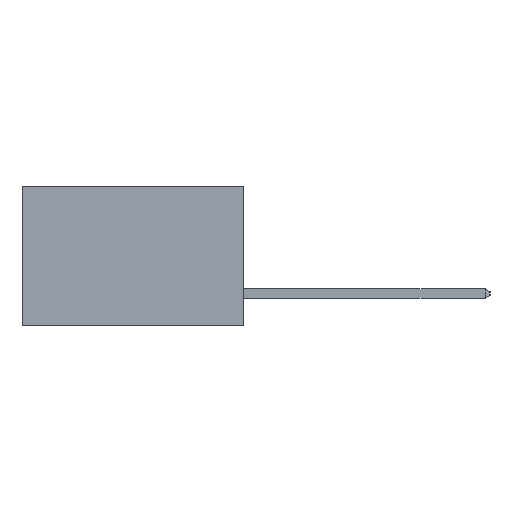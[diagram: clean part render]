
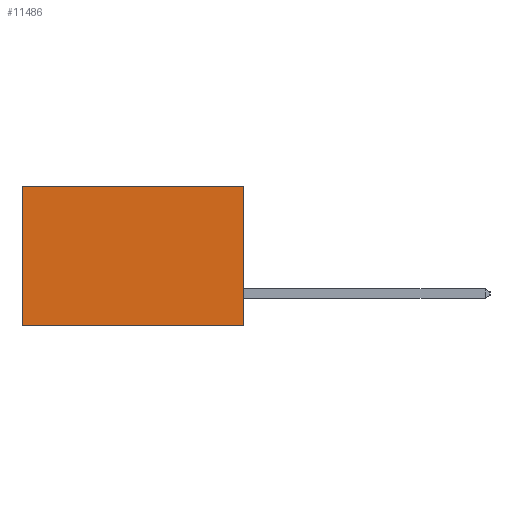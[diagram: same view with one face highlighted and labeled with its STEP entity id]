
A CAD part, left-side view. The second image highlights one B-rep face of the part: STEP entity #11486.
In plain terms, the highlighted planar face has unit normal (-1, 0, 0).
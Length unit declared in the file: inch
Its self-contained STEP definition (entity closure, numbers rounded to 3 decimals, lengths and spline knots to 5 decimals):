
#271 = DIRECTION ( 'NONE',  ( 1., 0., 0. ) ) ;
#1157 = ORIENTED_EDGE ( 'NONE', *, *, #2351, .F. ) ;
#1176 = CARTESIAN_POINT ( 'NONE',  ( 0.277, 0., 0. ) ) ;
#1626 = VERTEX_POINT ( 'NONE', #17747 ) ;
#2351 = EDGE_CURVE ( 'NONE', #14165, #17503, #17617, .T. ) ;
#2446 = EDGE_CURVE ( 'NONE', #15978, #1626, #14573, .T. ) ;
#3676 = PLANE ( 'NONE',  #7904 ) ;
#4421 = VECTOR ( 'NONE', #6976, 39.37008 ) ;
#5037 = ORIENTED_EDGE ( 'NONE', *, *, #11272, .T. ) ;
#6608 = CARTESIAN_POINT ( 'NONE',  ( 0.277, 0.59, -0.37 ) ) ;
#6827 = LINE ( 'NONE', #6608, #15629 ) ;
#6896 = CARTESIAN_POINT ( 'NONE',  ( 0.277, 0., -0.37 ) ) ;
#6922 = CARTESIAN_POINT ( 'NONE',  ( 0.277, 0., 0. ) ) ;
#6976 = DIRECTION ( 'NONE',  ( 0., 0., -1. ) ) ;
#7335 = DIRECTION ( 'NONE',  ( 0., 1., 0. ) ) ;
#7904 = AXIS2_PLACEMENT_3D ( 'NONE', #15373, #271, #17001 ) ;
#9593 = LINE ( 'NONE', #6896, #4421 ) ;
#10310 = VECTOR ( 'NONE', #7335, 39.37008 ) ;
#11073 = ORIENTED_EDGE ( 'NONE', *, *, #16235, .F. ) ;
#11080 = DIRECTION ( 'NONE',  ( 0., 1., 0. ) ) ;
#11272 = EDGE_CURVE ( 'NONE', #1626, #17503, #6827, .T. ) ;
#11486 = ADVANCED_FACE ( 'NONE', ( #19627 ), #3676, .F. ) ;
#11735 = ORIENTED_EDGE ( 'NONE', *, *, #2446, .T. ) ;
#12950 = EDGE_LOOP ( 'NONE', ( #5037, #1157, #11073, #11735 ) ) ;
#13505 = CARTESIAN_POINT ( 'NONE',  ( 0.277, 0.59, -0.37 ) ) ;
#14165 = VERTEX_POINT ( 'NONE', #19847 ) ;
#14573 = LINE ( 'NONE', #6922, #10310 ) ;
#15373 = CARTESIAN_POINT ( 'NONE',  ( 0.277, 0., -0.37 ) ) ;
#15629 = VECTOR ( 'NONE', #18112, 39.37008 ) ;
#15978 = VERTEX_POINT ( 'NONE', #1176 ) ;
#16235 = EDGE_CURVE ( 'NONE', #15978, #14165, #9593, .T. ) ;
#17001 = DIRECTION ( 'NONE',  ( 0., 0., -1. ) ) ;
#17115 = CARTESIAN_POINT ( 'NONE',  ( 0.277, 0., -0.37 ) ) ;
#17503 = VERTEX_POINT ( 'NONE', #13505 ) ;
#17617 = LINE ( 'NONE', #17115, #20354 ) ;
#17747 = CARTESIAN_POINT ( 'NONE',  ( 0.277, 0.59, 0. ) ) ;
#18112 = DIRECTION ( 'NONE',  ( 0., 0., -1. ) ) ;
#19627 = FACE_OUTER_BOUND ( 'NONE', #12950, .T. ) ;
#19847 = CARTESIAN_POINT ( 'NONE',  ( 0.277, 0., -0.37 ) ) ;
#20354 = VECTOR ( 'NONE', #11080, 39.37008 ) ;
